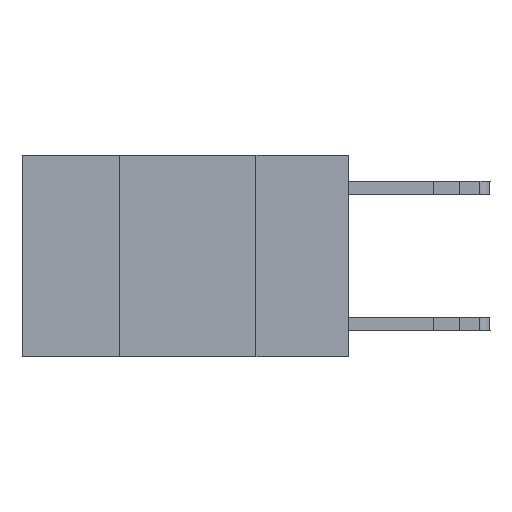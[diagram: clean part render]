
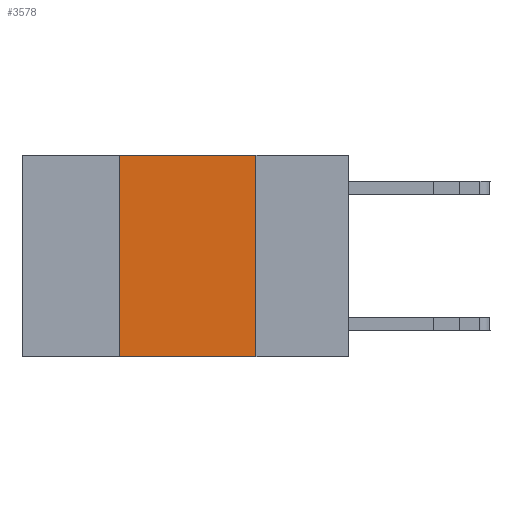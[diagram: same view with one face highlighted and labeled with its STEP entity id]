
A CAD part, left-side view. The second image highlights one B-rep face of the part: STEP entity #3578.
In plain terms, the highlighted planar face has unit normal (-1, 0, 0).
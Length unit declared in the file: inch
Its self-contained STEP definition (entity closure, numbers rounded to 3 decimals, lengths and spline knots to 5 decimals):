
#14 = VERTEX_POINT ( 'NONE', #12697 ) ;
#103 = DIRECTION ( 'NONE',  ( 0., 0., -1. ) ) ;
#1072 = CARTESIAN_POINT ( 'NONE',  ( 0., 0.17, -0.37 ) ) ;
#1257 = CARTESIAN_POINT ( 'NONE',  ( 0., 0.6, -0.37 ) ) ;
#1331 = VERTEX_POINT ( 'NONE', #6852 ) ;
#1847 = VERTEX_POINT ( 'NONE', #1072 ) ;
#2395 = VECTOR ( 'NONE', #103, 39.37008 ) ;
#2965 = VERTEX_POINT ( 'NONE', #12588 ) ;
#3137 = PLANE ( 'NONE',  #9659 ) ;
#3204 = CARTESIAN_POINT ( 'NONE',  ( 0., 0.17, 0. ) ) ;
#3578 = ADVANCED_FACE ( 'NONE', ( #11001 ), #3137, .F. ) ;
#4547 = VECTOR ( 'NONE', #5251, 39.37008 ) ;
#5251 = DIRECTION ( 'NONE',  ( 0., -1., 0. ) ) ;
#5555 = EDGE_LOOP ( 'NONE', ( #12211, #9661, #10686, #11020 ) ) ;
#6105 = EDGE_CURVE ( 'NONE', #14, #1847, #9039, .T. ) ;
#6852 = CARTESIAN_POINT ( 'NONE',  ( 0., 0.42, -0.37 ) ) ;
#6898 = LINE ( 'NONE', #7002, #7621 ) ;
#7002 = CARTESIAN_POINT ( 'NONE',  ( 0., 0.6, 0. ) ) ;
#7113 = DIRECTION ( 'NONE',  ( 1., 0., 0. ) ) ;
#7621 = VECTOR ( 'NONE', #11024, 39.37008 ) ;
#8154 = LINE ( 'NONE', #9318, #12865 ) ;
#8268 = EDGE_CURVE ( 'NONE', #1331, #1847, #11377, .T. ) ;
#8530 = EDGE_CURVE ( 'NONE', #2965, #14, #6898, .T. ) ;
#9039 = LINE ( 'NONE', #3204, #2395 ) ;
#9318 = CARTESIAN_POINT ( 'NONE',  ( 0., 0.42, 0. ) ) ;
#9390 = DIRECTION ( 'NONE',  ( 0., 0., 1. ) ) ;
#9659 = AXIS2_PLACEMENT_3D ( 'NONE', #10018, #7113, #11064 ) ;
#9661 = ORIENTED_EDGE ( 'NONE', *, *, #8530, .F. ) ;
#10018 = CARTESIAN_POINT ( 'NONE',  ( 0., 0.6, 0. ) ) ;
#10686 = ORIENTED_EDGE ( 'NONE', *, *, #11769, .F. ) ;
#11001 = FACE_OUTER_BOUND ( 'NONE', #5555, .T. ) ;
#11020 = ORIENTED_EDGE ( 'NONE', *, *, #8268, .T. ) ;
#11024 = DIRECTION ( 'NONE',  ( 0., -1., 0. ) ) ;
#11064 = DIRECTION ( 'NONE',  ( 0., 0., -1. ) ) ;
#11377 = LINE ( 'NONE', #1257, #4547 ) ;
#11769 = EDGE_CURVE ( 'NONE', #1331, #2965, #8154, .T. ) ;
#12211 = ORIENTED_EDGE ( 'NONE', *, *, #6105, .F. ) ;
#12588 = CARTESIAN_POINT ( 'NONE',  ( 0., 0.42, 0. ) ) ;
#12697 = CARTESIAN_POINT ( 'NONE',  ( 0., 0.17, 0. ) ) ;
#12865 = VECTOR ( 'NONE', #9390, 39.37008 ) ;
